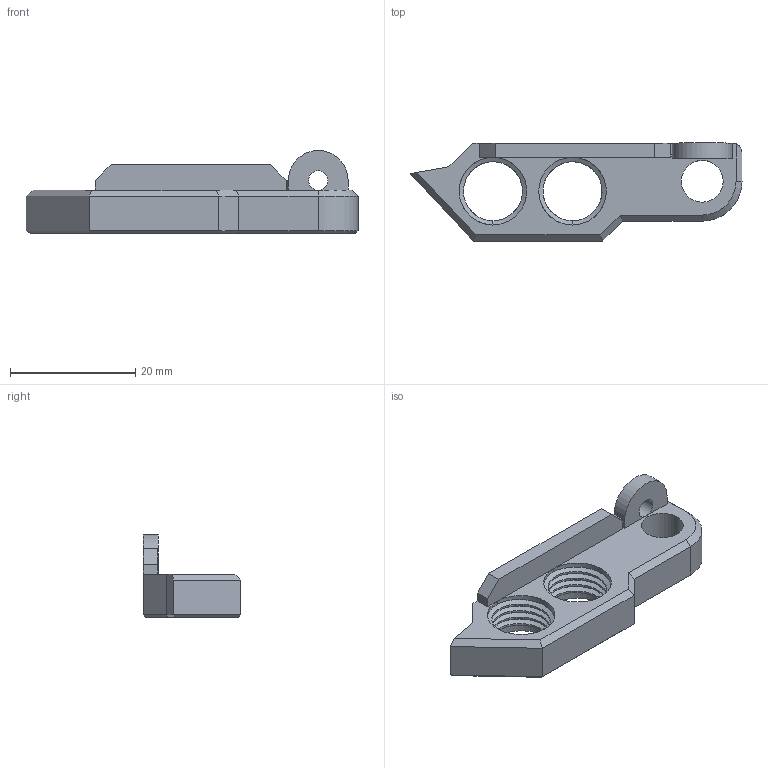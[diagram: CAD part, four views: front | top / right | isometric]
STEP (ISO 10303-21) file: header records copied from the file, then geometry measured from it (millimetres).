
FILE_DESCRIPTION (( 'STEP AP203' ), '1' );
FILE_NAME ('AF-HF-LR-PRT-004-STEP.STEP', '2020-10-04T16:08:40', ( '' ), ( '' ), 'SwSTEP 2.0', 'SolidWorks 2018', '' );
FILE_SCHEMA (( 'CONFIG_CONTROL_DESIGN' ));
Length unit declared in the file: inch
Products named in the file (1): AF-HF-LR-PRT-004-STEP
Bounding box: 52.99 x 15.62 x 13.23 mm (x, y, z)
Volume: 3534.2 mm3; surface area: 2902.4 mm2
Topology: 1 solids, 1 shells, 80 faces, 210 edges, 130 vertices
Faces by surface type: plane 41, cylinder 28, bspline 6, cone 5
Entity records: 3807 total; most frequent: CARTESIAN_POINT 1888, ORIENTED_EDGE 420, DIRECTION 343, EDGE_CURVE 210, VECTOR 133, LINE 133, VERTEX_POINT 130, AXIS2_PLACEMENT_3D 105
